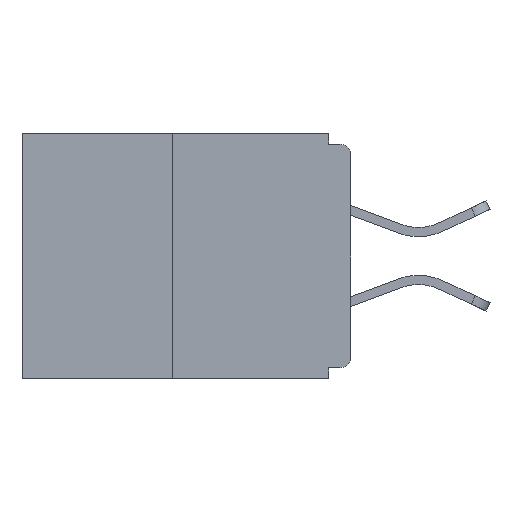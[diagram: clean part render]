
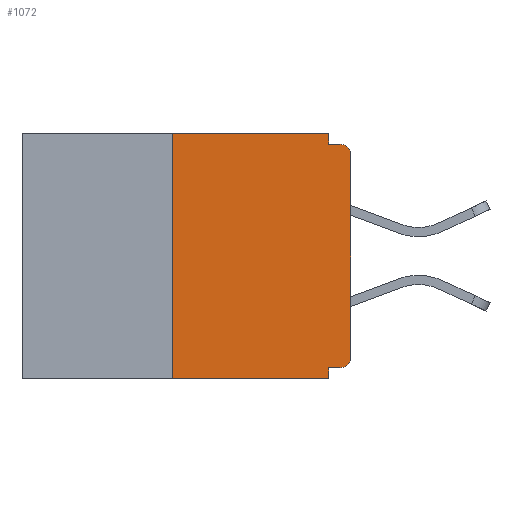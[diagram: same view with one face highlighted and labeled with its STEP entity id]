
A CAD part, left-side view. The second image highlights one B-rep face of the part: STEP entity #1072.
In plain terms, the highlighted planar face has unit normal (-1, 0, 0).
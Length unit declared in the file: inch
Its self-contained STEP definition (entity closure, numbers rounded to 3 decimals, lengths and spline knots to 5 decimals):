
#221 = LINE ( 'NONE', #12853, #1324 ) ;
#291 = LINE ( 'NONE', #18714, #30360 ) ;
#408 = VECTOR ( 'NONE', #3274, 39.37008 ) ;
#731 = CARTESIAN_POINT ( 'NONE',  ( 0., 0.031, 0. ) ) ;
#844 = DIRECTION ( 'NONE',  ( 0., -1., 0. ) ) ;
#1072 = ADVANCED_FACE ( 'NONE', ( #22654 ), #22424, .F. ) ;
#1078 = DIRECTION ( 'NONE',  ( 1., 0., 0. ) ) ;
#1324 = VECTOR ( 'NONE', #24594, 39.37008 ) ;
#2060 = LINE ( 'NONE', #15491, #29521 ) ;
#2640 = VERTEX_POINT ( 'NONE', #4929 ) ;
#2698 = VERTEX_POINT ( 'NONE', #14452 ) ;
#2804 = EDGE_CURVE ( 'NONE', #16110, #2698, #291, .T. ) ;
#3166 = DIRECTION ( 'NONE',  ( -1., 0., 0. ) ) ;
#3274 = DIRECTION ( 'NONE',  ( 0., -1., 0. ) ) ;
#3388 = DIRECTION ( 'NONE',  ( 0., 0., -1. ) ) ;
#4552 = EDGE_CURVE ( 'NONE', #5320, #4764, #18397, .T. ) ;
#4627 = ORIENTED_EDGE ( 'NONE', *, *, #2804, .F. ) ;
#4764 = VERTEX_POINT ( 'NONE', #26671 ) ;
#4929 = CARTESIAN_POINT ( 'NONE',  ( 0., 0.015, -0.328 ) ) ;
#5320 = VERTEX_POINT ( 'NONE', #11978 ) ;
#6020 = DIRECTION ( 'NONE',  ( 0., 0., -1. ) ) ;
#6105 = CARTESIAN_POINT ( 'NONE',  ( 0., 0.25, 0. ) ) ;
#6117 = VECTOR ( 'NONE', #10136, 39.37008 ) ;
#6961 = DIRECTION ( 'NONE',  ( 0., 0., -1. ) ) ;
#7763 = EDGE_CURVE ( 'NONE', #24291, #30113, #30115, .T. ) ;
#7798 = CARTESIAN_POINT ( 'NONE',  ( 0., 0.015, -0.313 ) ) ;
#7838 = CARTESIAN_POINT ( 'NONE',  ( 0., 0.015, -0.03 ) ) ;
#8245 = CARTESIAN_POINT ( 'NONE',  ( 0., 0., 0. ) ) ;
#8709 = LINE ( 'NONE', #731, #6117 ) ;
#9433 = CARTESIAN_POINT ( 'NONE',  ( 0., 0.015, -0.015 ) ) ;
#9610 = ORIENTED_EDGE ( 'NONE', *, *, #15841, .T. ) ;
#9897 = EDGE_CURVE ( 'NONE', #20984, #17180, #221, .T. ) ;
#10136 = DIRECTION ( 'NONE',  ( 0., 0., -1. ) ) ;
#10347 = EDGE_CURVE ( 'NONE', #2640, #16110, #27259, .T. ) ;
#11447 = DIRECTION ( 'NONE',  ( 0., 0., -1. ) ) ;
#11590 = ORIENTED_EDGE ( 'NONE', *, *, #9897, .F. ) ;
#11978 = CARTESIAN_POINT ( 'NONE',  ( 0., 0., -0.313 ) ) ;
#12853 = CARTESIAN_POINT ( 'NONE',  ( 0., 0.25, 0. ) ) ;
#12898 = CARTESIAN_POINT ( 'NONE',  ( 0., 0.031, -0.328 ) ) ;
#13454 = ORIENTED_EDGE ( 'NONE', *, *, #23161, .F. ) ;
#13780 = ORIENTED_EDGE ( 'NONE', *, *, #7763, .F. ) ;
#14452 = CARTESIAN_POINT ( 'NONE',  ( 0., 0.031, -0.343 ) ) ;
#14650 = CIRCLE ( 'NONE', #26511, 0.015 ) ;
#15491 = CARTESIAN_POINT ( 'NONE',  ( 0., 0.46, -0.343 ) ) ;
#15841 = EDGE_CURVE ( 'NONE', #4764, #30113, #14650, .T. ) ;
#16110 = VERTEX_POINT ( 'NONE', #12898 ) ;
#16252 = EDGE_CURVE ( 'NONE', #20984, #2698, #2060, .T. ) ;
#16775 = CARTESIAN_POINT ( 'NONE',  ( 0., 0., -0.328 ) ) ;
#17147 = DIRECTION ( 'NONE',  ( -1., 0., 0. ) ) ;
#17180 = VERTEX_POINT ( 'NONE', #6105 ) ;
#17837 = EDGE_CURVE ( 'NONE', #2640, #5320, #25555, .T. ) ;
#18397 = LINE ( 'NONE', #8245, #26181 ) ;
#18714 = CARTESIAN_POINT ( 'NONE',  ( 0., 0.031, -0.343 ) ) ;
#19814 = VECTOR ( 'NONE', #28907, 39.37008 ) ;
#19959 = ORIENTED_EDGE ( 'NONE', *, *, #17837, .T. ) ;
#20268 = AXIS2_PLACEMENT_3D ( 'NONE', #25225, #1078, #6020 ) ;
#20639 = AXIS2_PLACEMENT_3D ( 'NONE', #7798, #17147, #6961 ) ;
#20984 = VERTEX_POINT ( 'NONE', #26476 ) ;
#22424 = PLANE ( 'NONE',  #20268 ) ;
#22654 = FACE_OUTER_BOUND ( 'NONE', #29765, .T. ) ;
#22705 = CARTESIAN_POINT ( 'NONE',  ( 0., 0.46, 0. ) ) ;
#22896 = VECTOR ( 'NONE', #844, 39.37008 ) ;
#23161 = EDGE_CURVE ( 'NONE', #17180, #25817, #29956, .T. ) ;
#23892 = EDGE_CURVE ( 'NONE', #25817, #24291, #8709, .T. ) ;
#23996 = ORIENTED_EDGE ( 'NONE', *, *, #4552, .T. ) ;
#24057 = ORIENTED_EDGE ( 'NONE', *, *, #16252, .T. ) ;
#24291 = VERTEX_POINT ( 'NONE', #25587 ) ;
#24594 = DIRECTION ( 'NONE',  ( 0., 0., 1. ) ) ;
#25225 = CARTESIAN_POINT ( 'NONE',  ( 0., 0.46, 0. ) ) ;
#25253 = DIRECTION ( 'NONE',  ( 0., -1., 0. ) ) ;
#25389 = ORIENTED_EDGE ( 'NONE', *, *, #10347, .F. ) ;
#25555 = CIRCLE ( 'NONE', #20639, 0.015 ) ;
#25575 = CARTESIAN_POINT ( 'NONE',  ( 0., 0.031, 0. ) ) ;
#25587 = CARTESIAN_POINT ( 'NONE',  ( 0., 0.031, -0.015 ) ) ;
#25817 = VERTEX_POINT ( 'NONE', #25575 ) ;
#26181 = VECTOR ( 'NONE', #29527, 39.37008 ) ;
#26476 = CARTESIAN_POINT ( 'NONE',  ( 0., 0.25, -0.343 ) ) ;
#26511 = AXIS2_PLACEMENT_3D ( 'NONE', #7838, #3166, #3388 ) ;
#26671 = CARTESIAN_POINT ( 'NONE',  ( 0., 0., -0.03 ) ) ;
#27259 = LINE ( 'NONE', #16775, #19814 ) ;
#28003 = ORIENTED_EDGE ( 'NONE', *, *, #23892, .F. ) ;
#28907 = DIRECTION ( 'NONE',  ( 0., 1., 0. ) ) ;
#29333 = CARTESIAN_POINT ( 'NONE',  ( 0., 0., -0.015 ) ) ;
#29521 = VECTOR ( 'NONE', #25253, 39.37008 ) ;
#29527 = DIRECTION ( 'NONE',  ( 0., 0., 1. ) ) ;
#29765 = EDGE_LOOP ( 'NONE', ( #13454, #11590, #24057, #4627, #25389, #19959, #23996, #9610, #13780, #28003 ) ) ;
#29956 = LINE ( 'NONE', #22705, #22896 ) ;
#30113 = VERTEX_POINT ( 'NONE', #9433 ) ;
#30115 = LINE ( 'NONE', #29333, #408 ) ;
#30360 = VECTOR ( 'NONE', #11447, 39.37008 ) ;
